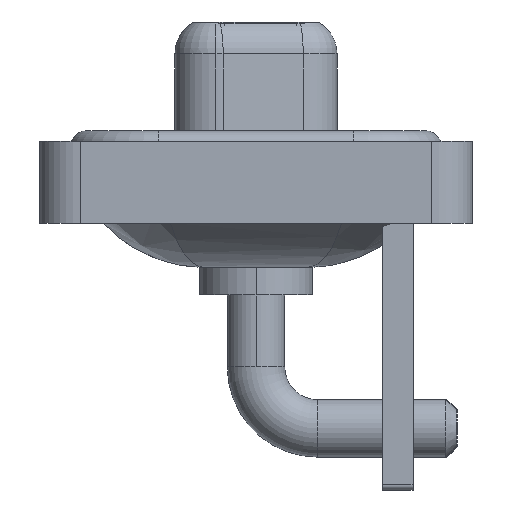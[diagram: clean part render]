
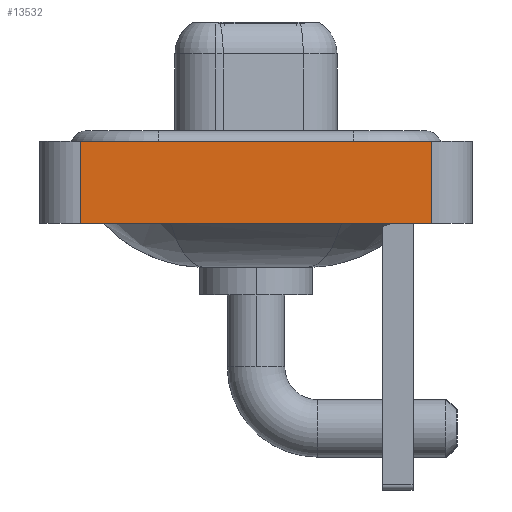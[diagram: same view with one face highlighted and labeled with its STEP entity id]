
A CAD part, left-side view. The second image highlights one B-rep face of the part: STEP entity #13532.
In plain terms, the highlighted planar face has unit normal (-1, 0, 0).
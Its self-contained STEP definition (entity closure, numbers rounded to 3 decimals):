
#310 = CARTESIAN_POINT ( 'NONE',  ( -7.25, -8.55, -3.6 ) ) ;
#497 = DIRECTION ( 'NONE',  ( 0., 0., 1. ) ) ;
#1551 = CARTESIAN_POINT ( 'NONE',  ( -7.25, 8.55, 0.4 ) ) ;
#2541 = CARTESIAN_POINT ( 'NONE',  ( -7.25, -8.55, 0.4 ) ) ;
#2544 = EDGE_CURVE ( 'NONE', #9056, #3343, #12882, .T. ) ;
#2881 = VERTEX_POINT ( 'NONE', #1551 ) ;
#3343 = VERTEX_POINT ( 'NONE', #3558 ) ;
#3558 = CARTESIAN_POINT ( 'NONE',  ( -7.25, -8.55, 0.4 ) ) ;
#4124 = DIRECTION ( 'NONE',  ( -1., 0., 0. ) ) ;
#4407 = EDGE_CURVE ( 'NONE', #9813, #2881, #6445, .T. ) ;
#5076 = EDGE_LOOP ( 'NONE', ( #6024, #9413, #10597, #16798 ) ) ;
#5419 = CARTESIAN_POINT ( 'NONE',  ( -7.25, -8.55, -3.6 ) ) ;
#5482 = FACE_OUTER_BOUND ( 'NONE', #5076, .T. ) ;
#6024 = ORIENTED_EDGE ( 'NONE', *, *, #2544, .T. ) ;
#6247 = AXIS2_PLACEMENT_3D ( 'NONE', #16400, #4124, #9585 ) ;
#6262 = VECTOR ( 'NONE', #14590, 1000. ) ;
#6445 = LINE ( 'NONE', #10582, #6262 ) ;
#7099 = CARTESIAN_POINT ( 'NONE',  ( -7.25, 8.55, -3.6 ) ) ;
#7153 = VECTOR ( 'NONE', #497, 1000. ) ;
#9056 = VERTEX_POINT ( 'NONE', #310 ) ;
#9191 = DIRECTION ( 'NONE',  ( 0., -1., 0. ) ) ;
#9413 = ORIENTED_EDGE ( 'NONE', *, *, #16695, .F. ) ;
#9585 = DIRECTION ( 'NONE',  ( 0., 0., 1. ) ) ;
#9692 = VECTOR ( 'NONE', #10707, 1000. ) ;
#9813 = VERTEX_POINT ( 'NONE', #7099 ) ;
#10220 = VECTOR ( 'NONE', #9191, 1000. ) ;
#10582 = CARTESIAN_POINT ( 'NONE',  ( -7.25, 8.55, -3.6 ) ) ;
#10597 = ORIENTED_EDGE ( 'NONE', *, *, #4407, .F. ) ;
#10621 = LINE ( 'NONE', #5419, #9692 ) ;
#10707 = DIRECTION ( 'NONE',  ( 0., -1., 0. ) ) ;
#10947 = PLANE ( 'NONE',  #6247 ) ;
#12882 = LINE ( 'NONE', #17004, #7153 ) ;
#13532 = ADVANCED_FACE ( 'NONE', ( #5482 ), #10947, .T. ) ;
#14590 = DIRECTION ( 'NONE',  ( 0., 0., 1. ) ) ;
#15285 = EDGE_CURVE ( 'NONE', #9813, #9056, #10621, .T. ) ;
#15977 = LINE ( 'NONE', #2541, #10220 ) ;
#16400 = CARTESIAN_POINT ( 'NONE',  ( -7.25, -8.55, -3.6 ) ) ;
#16695 = EDGE_CURVE ( 'NONE', #2881, #3343, #15977, .T. ) ;
#16798 = ORIENTED_EDGE ( 'NONE', *, *, #15285, .T. ) ;
#17004 = CARTESIAN_POINT ( 'NONE',  ( -7.25, -8.55, -3.6 ) ) ;
